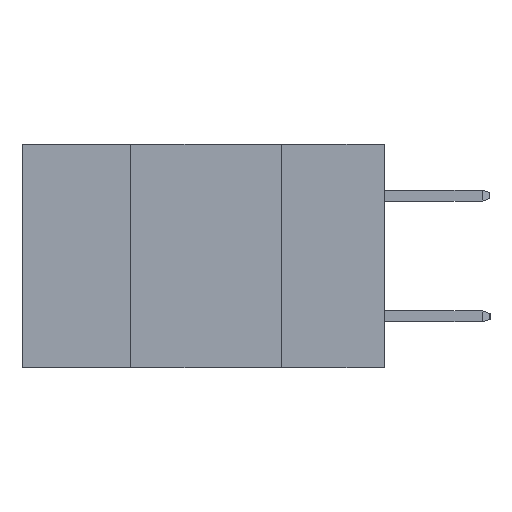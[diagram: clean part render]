
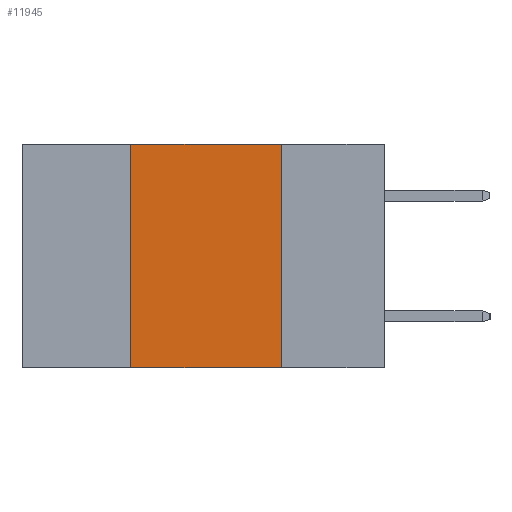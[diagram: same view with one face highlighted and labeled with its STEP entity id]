
A CAD part, left-side view. The second image highlights one B-rep face of the part: STEP entity #11945.
In plain terms, the highlighted planar face has unit normal (-1, 0, 0).
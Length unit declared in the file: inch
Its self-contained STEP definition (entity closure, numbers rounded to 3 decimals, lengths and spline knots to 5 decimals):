
#346 = CARTESIAN_POINT ( 'NONE',  ( 0., 0.17, -0.37 ) ) ;
#521 = EDGE_CURVE ( 'NONE', #6573, #6890, #5149, .T. ) ;
#1513 = VECTOR ( 'NONE', #8528, 39.37008 ) ;
#1627 = DIRECTION ( 'NONE',  ( 0., 0., 1. ) ) ;
#2564 = EDGE_CURVE ( 'NONE', #6573, #3051, #9508, .T. ) ;
#2676 = VECTOR ( 'NONE', #6882, 39.37008 ) ;
#2690 = CARTESIAN_POINT ( 'NONE',  ( 0., 0.42, -0.37 ) ) ;
#2840 = EDGE_CURVE ( 'NONE', #4854, #3051, #11342, .T. ) ;
#3051 = VERTEX_POINT ( 'NONE', #346 ) ;
#3599 = CARTESIAN_POINT ( 'NONE',  ( 0., 0.6, 0. ) ) ;
#4216 = EDGE_CURVE ( 'NONE', #6890, #4854, #12485, .T. ) ;
#4549 = AXIS2_PLACEMENT_3D ( 'NONE', #3599, #10440, #4619 ) ;
#4557 = CARTESIAN_POINT ( 'NONE',  ( 0., 0.42, -0.37 ) ) ;
#4619 = DIRECTION ( 'NONE',  ( 0., 0., -1. ) ) ;
#4741 = CARTESIAN_POINT ( 'NONE',  ( 0., 0.17, -0.37 ) ) ;
#4821 = DIRECTION ( 'NONE',  ( 0., 0., -1. ) ) ;
#4854 = VERTEX_POINT ( 'NONE', #7165 ) ;
#5130 = CARTESIAN_POINT ( 'NONE',  ( 0., 0.42, 0. ) ) ;
#5149 = LINE ( 'NONE', #4557, #9987 ) ;
#5654 = ORIENTED_EDGE ( 'NONE', *, *, #521, .F. ) ;
#6175 = VECTOR ( 'NONE', #4821, 39.37008 ) ;
#6251 = ORIENTED_EDGE ( 'NONE', *, *, #4216, .F. ) ;
#6573 = VERTEX_POINT ( 'NONE', #2690 ) ;
#6862 = ORIENTED_EDGE ( 'NONE', *, *, #2564, .T. ) ;
#6882 = DIRECTION ( 'NONE',  ( 0., -1., 0. ) ) ;
#6890 = VERTEX_POINT ( 'NONE', #5130 ) ;
#7165 = CARTESIAN_POINT ( 'NONE',  ( 0., 0.17, 0. ) ) ;
#8022 = FACE_OUTER_BOUND ( 'NONE', #10326, .T. ) ;
#8246 = CARTESIAN_POINT ( 'NONE',  ( 0., 0.6, 0. ) ) ;
#8506 = PLANE ( 'NONE',  #4549 ) ;
#8528 = DIRECTION ( 'NONE',  ( 0., -1., 0. ) ) ;
#8954 = CARTESIAN_POINT ( 'NONE',  ( 0., 0.6, -0.37 ) ) ;
#9508 = LINE ( 'NONE', #8954, #1513 ) ;
#9987 = VECTOR ( 'NONE', #1627, 39.37008 ) ;
#10326 = EDGE_LOOP ( 'NONE', ( #12458, #6251, #5654, #6862 ) ) ;
#10440 = DIRECTION ( 'NONE',  ( 1., 0., 0. ) ) ;
#11342 = LINE ( 'NONE', #4741, #6175 ) ;
#11945 = ADVANCED_FACE ( 'NONE', ( #8022 ), #8506, .F. ) ;
#12458 = ORIENTED_EDGE ( 'NONE', *, *, #2840, .F. ) ;
#12485 = LINE ( 'NONE', #8246, #2676 ) ;
